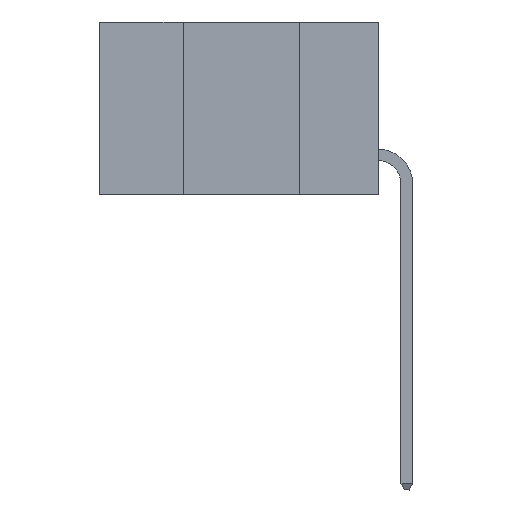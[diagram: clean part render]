
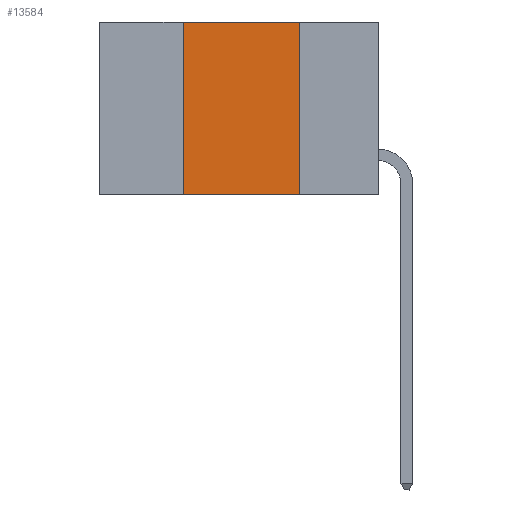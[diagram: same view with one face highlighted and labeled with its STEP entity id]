
A CAD part, left-side view. The second image highlights one B-rep face of the part: STEP entity #13584.
In plain terms, the highlighted planar face has unit normal (-1, 0, 0).
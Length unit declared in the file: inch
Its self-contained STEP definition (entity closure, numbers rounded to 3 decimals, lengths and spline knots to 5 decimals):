
#260 = DIRECTION ( 'NONE',  ( 0., 0., -1. ) ) ;
#301 = EDGE_CURVE ( 'NONE', #11907, #19110, #19956, .T. ) ;
#928 = CARTESIAN_POINT ( 'NONE',  ( 0., 0.6, -0.37 ) ) ;
#1145 = EDGE_CURVE ( 'NONE', #5568, #21526, #16215, .T. ) ;
#1925 = CARTESIAN_POINT ( 'NONE',  ( 0., 0.42, -0.37 ) ) ;
#2146 = EDGE_CURVE ( 'NONE', #19110, #21526, #5275, .T. ) ;
#3388 = EDGE_CURVE ( 'NONE', #5568, #11907, #15227, .T. ) ;
#4782 = VECTOR ( 'NONE', #260, 39.37008 ) ;
#5055 = CARTESIAN_POINT ( 'NONE',  ( 0., 0.17, -0.37 ) ) ;
#5275 = LINE ( 'NONE', #5055, #4782 ) ;
#5478 = VECTOR ( 'NONE', #6381, 39.37008 ) ;
#5568 = VERTEX_POINT ( 'NONE', #20669 ) ;
#6102 = DIRECTION ( 'NONE',  ( 1., 0., 0. ) ) ;
#6381 = DIRECTION ( 'NONE',  ( 0., -1., 0. ) ) ;
#6441 = FACE_OUTER_BOUND ( 'NONE', #16725, .T. ) ;
#7303 = CARTESIAN_POINT ( 'NONE',  ( 0., 0.17, 0. ) ) ;
#8333 = CARTESIAN_POINT ( 'NONE',  ( 0., 0.6, 0. ) ) ;
#9013 = CARTESIAN_POINT ( 'NONE',  ( 0., 0.17, -0.37 ) ) ;
#9701 = DIRECTION ( 'NONE',  ( 0., 0., -1. ) ) ;
#11088 = ORIENTED_EDGE ( 'NONE', *, *, #1145, .T. ) ;
#11263 = ORIENTED_EDGE ( 'NONE', *, *, #2146, .F. ) ;
#11634 = AXIS2_PLACEMENT_3D ( 'NONE', #13026, #6102, #9701 ) ;
#11907 = VERTEX_POINT ( 'NONE', #18085 ) ;
#12558 = ORIENTED_EDGE ( 'NONE', *, *, #301, .F. ) ;
#13026 = CARTESIAN_POINT ( 'NONE',  ( 0., 0.6, 0. ) ) ;
#13584 = ADVANCED_FACE ( 'NONE', ( #6441 ), #14702, .F. ) ;
#14702 = PLANE ( 'NONE',  #11634 ) ;
#15227 = LINE ( 'NONE', #1925, #19468 ) ;
#16215 = LINE ( 'NONE', #928, #5478 ) ;
#16725 = EDGE_LOOP ( 'NONE', ( #11263, #12558, #16880, #11088 ) ) ;
#16880 = ORIENTED_EDGE ( 'NONE', *, *, #3388, .F. ) ;
#18085 = CARTESIAN_POINT ( 'NONE',  ( 0., 0.42, 0. ) ) ;
#19110 = VERTEX_POINT ( 'NONE', #7303 ) ;
#19468 = VECTOR ( 'NONE', #22039, 39.37008 ) ;
#19956 = LINE ( 'NONE', #8333, #21841 ) ;
#20168 = DIRECTION ( 'NONE',  ( 0., -1., 0. ) ) ;
#20669 = CARTESIAN_POINT ( 'NONE',  ( 0., 0.42, -0.37 ) ) ;
#21526 = VERTEX_POINT ( 'NONE', #9013 ) ;
#21841 = VECTOR ( 'NONE', #20168, 39.37008 ) ;
#22039 = DIRECTION ( 'NONE',  ( 0., 0., 1. ) ) ;
